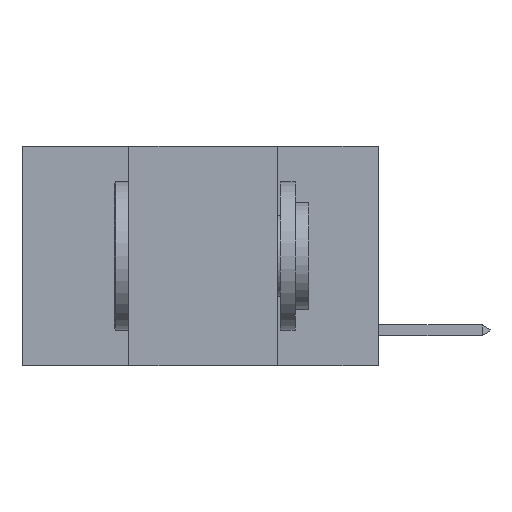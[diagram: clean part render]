
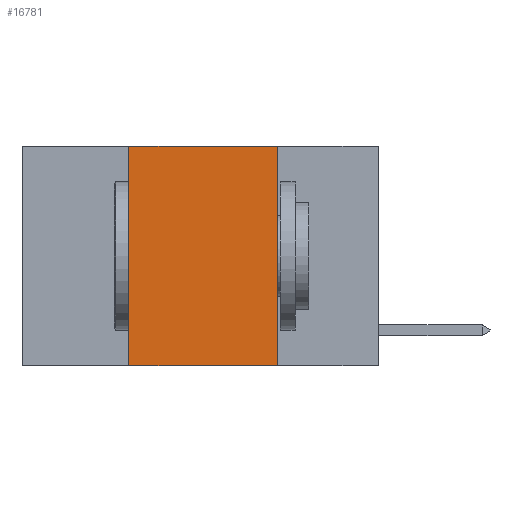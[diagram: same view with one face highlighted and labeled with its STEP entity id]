
A CAD part, left-side view. The second image highlights one B-rep face of the part: STEP entity #16781.
In plain terms, the highlighted planar face has unit normal (-1, 0, 0).
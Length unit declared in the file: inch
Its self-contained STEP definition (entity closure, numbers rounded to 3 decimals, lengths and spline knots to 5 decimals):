
#169 = VERTEX_POINT ( 'NONE', #16927 ) ;
#470 = DIRECTION ( 'NONE',  ( 0., 0., -1. ) ) ;
#1401 = CARTESIAN_POINT ( 'NONE',  ( 0., 0.6, -0.37 ) ) ;
#3288 = DIRECTION ( 'NONE',  ( 0., -1., 0. ) ) ;
#3789 = CARTESIAN_POINT ( 'NONE',  ( 0., 0.17, 0. ) ) ;
#3901 = VERTEX_POINT ( 'NONE', #3789 ) ;
#4144 = LINE ( 'NONE', #1401, #7852 ) ;
#5462 = ORIENTED_EDGE ( 'NONE', *, *, #17392, .F. ) ;
#6879 = EDGE_CURVE ( 'NONE', #10952, #169, #12741, .T. ) ;
#7595 = VECTOR ( 'NONE', #13696, 39.37008 ) ;
#7852 = VECTOR ( 'NONE', #3288, 39.37008 ) ;
#8168 = VERTEX_POINT ( 'NONE', #15474 ) ;
#9790 = PLANE ( 'NONE',  #23362 ) ;
#9931 = CARTESIAN_POINT ( 'NONE',  ( 0., 0.42, 0. ) ) ;
#10952 = VERTEX_POINT ( 'NONE', #20761 ) ;
#11312 = CARTESIAN_POINT ( 'NONE',  ( 0., 0.6, 0. ) ) ;
#11385 = DIRECTION ( 'NONE',  ( 0., 0., -1. ) ) ;
#11575 = EDGE_CURVE ( 'NONE', #3901, #8168, #23045, .T. ) ;
#11971 = LINE ( 'NONE', #15968, #13140 ) ;
#12278 = FACE_OUTER_BOUND ( 'NONE', #17721, .T. ) ;
#12741 = LINE ( 'NONE', #9931, #7595 ) ;
#13140 = VECTOR ( 'NONE', #21111, 39.37008 ) ;
#13179 = DIRECTION ( 'NONE',  ( 1., 0., 0. ) ) ;
#13696 = DIRECTION ( 'NONE',  ( 0., 0., 1. ) ) ;
#14973 = CARTESIAN_POINT ( 'NONE',  ( 0., 0.17, 0. ) ) ;
#14983 = ORIENTED_EDGE ( 'NONE', *, *, #6879, .F. ) ;
#15474 = CARTESIAN_POINT ( 'NONE',  ( 0., 0.17, -0.37 ) ) ;
#15968 = CARTESIAN_POINT ( 'NONE',  ( 0., 0.6, 0. ) ) ;
#16781 = ADVANCED_FACE ( 'NONE', ( #12278 ), #9790, .F. ) ;
#16927 = CARTESIAN_POINT ( 'NONE',  ( 0., 0.42, 0. ) ) ;
#17392 = EDGE_CURVE ( 'NONE', #169, #3901, #11971, .T. ) ;
#17674 = VECTOR ( 'NONE', #11385, 39.37008 ) ;
#17721 = EDGE_LOOP ( 'NONE', ( #19950, #5462, #14983, #23564 ) ) ;
#19520 = EDGE_CURVE ( 'NONE', #10952, #8168, #4144, .T. ) ;
#19950 = ORIENTED_EDGE ( 'NONE', *, *, #11575, .F. ) ;
#20761 = CARTESIAN_POINT ( 'NONE',  ( 0., 0.42, -0.37 ) ) ;
#21111 = DIRECTION ( 'NONE',  ( 0., -1., 0. ) ) ;
#23045 = LINE ( 'NONE', #14973, #17674 ) ;
#23362 = AXIS2_PLACEMENT_3D ( 'NONE', #11312, #13179, #470 ) ;
#23564 = ORIENTED_EDGE ( 'NONE', *, *, #19520, .T. ) ;
